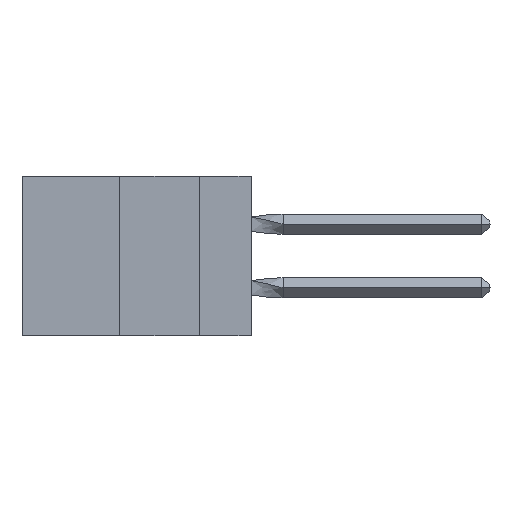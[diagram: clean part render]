
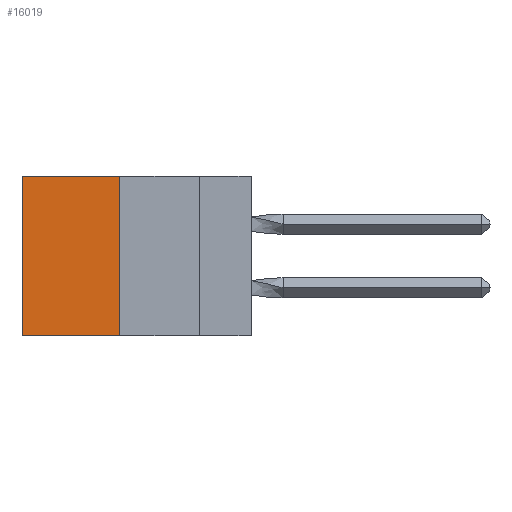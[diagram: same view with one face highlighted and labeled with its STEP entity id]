
A CAD part, left-side view. The second image highlights one B-rep face of the part: STEP entity #16019.
In plain terms, the highlighted planar face has unit normal (-1, 0, 0).
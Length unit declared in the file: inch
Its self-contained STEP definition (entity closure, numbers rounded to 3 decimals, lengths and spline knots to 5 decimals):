
#79 = VERTEX_POINT ( 'NONE', #4507 ) ;
#171 = CARTESIAN_POINT ( 'NONE',  ( 0.305, 0.413, -0.5 ) ) ;
#417 = ORIENTED_EDGE ( 'NONE', *, *, #10287, .T. ) ;
#507 = CARTESIAN_POINT ( 'NONE',  ( 0.305, 0.413, -0.5 ) ) ;
#774 = FACE_OUTER_BOUND ( 'NONE', #2013, .T. ) ;
#1125 = LINE ( 'NONE', #2144, #7511 ) ;
#2013 = EDGE_LOOP ( 'NONE', ( #15781, #14399, #4486, #417 ) ) ;
#2144 = CARTESIAN_POINT ( 'NONE',  ( 0.305, 0.72, -0.5 ) ) ;
#3126 = VECTOR ( 'NONE', #8238, 39.37008 ) ;
#3778 = CARTESIAN_POINT ( 'NONE',  ( 0.305, 0.72, 0. ) ) ;
#4486 = ORIENTED_EDGE ( 'NONE', *, *, #17065, .F. ) ;
#4507 = CARTESIAN_POINT ( 'NONE',  ( 0.305, 0.72, -0.5 ) ) ;
#5506 = CARTESIAN_POINT ( 'NONE',  ( 0.305, 0.413, 0. ) ) ;
#5673 = CARTESIAN_POINT ( 'NONE',  ( 0.305, 0.413, -0.5 ) ) ;
#6180 = DIRECTION ( 'NONE',  ( 0., 0., -1. ) ) ;
#6579 = CARTESIAN_POINT ( 'NONE',  ( 0.305, 0.413, -0.5 ) ) ;
#7254 = EDGE_CURVE ( 'NONE', #15044, #79, #1125, .T. ) ;
#7511 = VECTOR ( 'NONE', #6180, 39.37008 ) ;
#8190 = VECTOR ( 'NONE', #14037, 39.37008 ) ;
#8238 = DIRECTION ( 'NONE',  ( 0., 1., 0. ) ) ;
#8290 = DIRECTION ( 'NONE',  ( 0., 1., 0. ) ) ;
#8630 = LINE ( 'NONE', #5673, #16708 ) ;
#8870 = LINE ( 'NONE', #5506, #3126 ) ;
#9171 = AXIS2_PLACEMENT_3D ( 'NONE', #6579, #12014, #14644 ) ;
#10287 = EDGE_CURVE ( 'NONE', #13387, #15044, #8870, .T. ) ;
#11776 = LINE ( 'NONE', #507, #8190 ) ;
#11844 = PLANE ( 'NONE',  #9171 ) ;
#12014 = DIRECTION ( 'NONE',  ( 1., 0., 0. ) ) ;
#13387 = VERTEX_POINT ( 'NONE', #16888 ) ;
#14037 = DIRECTION ( 'NONE',  ( 0., 0., -1. ) ) ;
#14399 = ORIENTED_EDGE ( 'NONE', *, *, #16971, .F. ) ;
#14644 = DIRECTION ( 'NONE',  ( 0., 0., -1. ) ) ;
#14706 = VERTEX_POINT ( 'NONE', #171 ) ;
#15044 = VERTEX_POINT ( 'NONE', #3778 ) ;
#15781 = ORIENTED_EDGE ( 'NONE', *, *, #7254, .T. ) ;
#16019 = ADVANCED_FACE ( 'NONE', ( #774 ), #11844, .F. ) ;
#16708 = VECTOR ( 'NONE', #8290, 39.37008 ) ;
#16888 = CARTESIAN_POINT ( 'NONE',  ( 0.305, 0.413, 0. ) ) ;
#16971 = EDGE_CURVE ( 'NONE', #14706, #79, #8630, .T. ) ;
#17065 = EDGE_CURVE ( 'NONE', #13387, #14706, #11776, .T. ) ;
